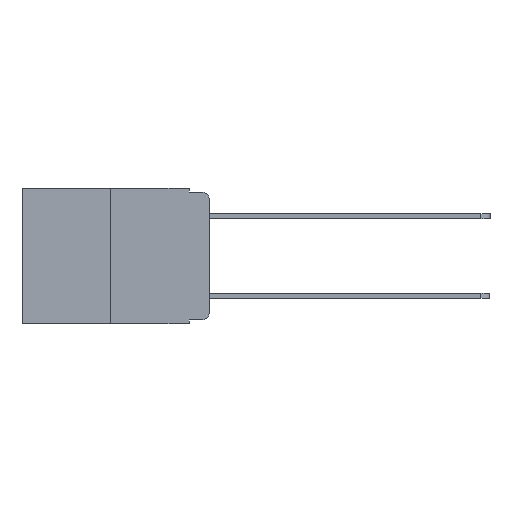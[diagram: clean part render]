
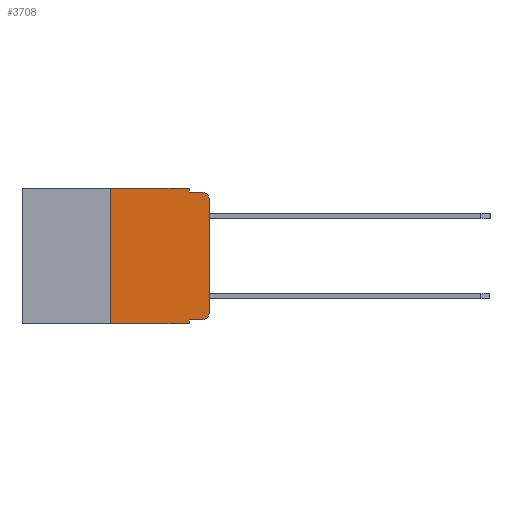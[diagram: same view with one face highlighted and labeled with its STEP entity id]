
A CAD part, left-side view. The second image highlights one B-rep face of the part: STEP entity #3708.
In plain terms, the highlighted planar face has unit normal (-1, 0, 0).
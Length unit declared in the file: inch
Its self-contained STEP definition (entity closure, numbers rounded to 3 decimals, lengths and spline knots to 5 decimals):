
#12 = EDGE_CURVE ( 'NONE', #16790, #11904, #22205, .T. ) ;
#94 = CARTESIAN_POINT ( 'NONE',  ( 0., 0., -0.313 ) ) ;
#160 = FACE_OUTER_BOUND ( 'NONE', #13219, .T. ) ;
#509 = EDGE_CURVE ( 'NONE', #11904, #1297, #18472, .T. ) ;
#678 = DIRECTION ( 'NONE',  ( 0., 0., -1. ) ) ;
#687 = CARTESIAN_POINT ( 'NONE',  ( 0., 0.25, 0. ) ) ;
#1297 = VERTEX_POINT ( 'NONE', #94 ) ;
#1378 = CARTESIAN_POINT ( 'NONE',  ( 0., 0.02, -0.01 ) ) ;
#1591 = ORIENTED_EDGE ( 'NONE', *, *, #10292, .T. ) ;
#1808 = CARTESIAN_POINT ( 'NONE',  ( 0., 0.473, 0. ) ) ;
#3054 = CARTESIAN_POINT ( 'NONE',  ( 0., 0.051, 0. ) ) ;
#3351 = CARTESIAN_POINT ( 'NONE',  ( 0., 0.051, -0.343 ) ) ;
#3483 = VECTOR ( 'NONE', #13661, 39.37008 ) ;
#3509 = DIRECTION ( 'NONE',  ( 0., 0., -1. ) ) ;
#3539 = DIRECTION ( 'NONE',  ( -1., 0., 0. ) ) ;
#3667 = CARTESIAN_POINT ( 'NONE',  ( 0., 0.051, 0. ) ) ;
#3708 = ADVANCED_FACE ( 'NONE', ( #160 ), #17959, .F. ) ;
#3719 = DIRECTION ( 'NONE',  ( 0., -1., 0. ) ) ;
#4081 = LINE ( 'NONE', #687, #3483 ) ;
#4088 = LINE ( 'NONE', #3054, #18382 ) ;
#4102 = LINE ( 'NONE', #4581, #22365 ) ;
#4274 = ORIENTED_EDGE ( 'NONE', *, *, #8604, .F. ) ;
#4296 = DIRECTION ( 'NONE',  ( 0., -1., 0. ) ) ;
#4581 = CARTESIAN_POINT ( 'NONE',  ( 0., 0., 0. ) ) ;
#5077 = CARTESIAN_POINT ( 'NONE',  ( 0., 0.051, -0.333 ) ) ;
#5721 = ORIENTED_EDGE ( 'NONE', *, *, #20432, .T. ) ;
#5916 = EDGE_CURVE ( 'NONE', #13882, #7065, #23062, .T. ) ;
#6126 = CARTESIAN_POINT ( 'NONE',  ( 0., 0.25, -0.343 ) ) ;
#6276 = VECTOR ( 'NONE', #10702, 39.37008 ) ;
#7065 = VERTEX_POINT ( 'NONE', #3667 ) ;
#7349 = DIRECTION ( 'NONE',  ( 0., 0., -1. ) ) ;
#7488 = ORIENTED_EDGE ( 'NONE', *, *, #13862, .T. ) ;
#7541 = VERTEX_POINT ( 'NONE', #15515 ) ;
#8204 = CARTESIAN_POINT ( 'NONE',  ( 0., 0.25, 0. ) ) ;
#8300 = VECTOR ( 'NONE', #21865, 39.37008 ) ;
#8604 = EDGE_CURVE ( 'NONE', #7065, #7541, #4088, .T. ) ;
#9168 = CARTESIAN_POINT ( 'NONE',  ( 0., 0.473, 0. ) ) ;
#9256 = ORIENTED_EDGE ( 'NONE', *, *, #5916, .F. ) ;
#9289 = VECTOR ( 'NONE', #3719, 39.37008 ) ;
#9515 = LINE ( 'NONE', #15171, #18799 ) ;
#10292 = EDGE_CURVE ( 'NONE', #20953, #23064, #9515, .T. ) ;
#10702 = DIRECTION ( 'NONE',  ( 0., -1., 0. ) ) ;
#11309 = AXIS2_PLACEMENT_3D ( 'NONE', #22149, #11958, #678 ) ;
#11904 = VERTEX_POINT ( 'NONE', #21791 ) ;
#11958 = DIRECTION ( 'NONE',  ( -1., 0., 0. ) ) ;
#12149 = DIRECTION ( 'NONE',  ( 0., 0., 1. ) ) ;
#12350 = CARTESIAN_POINT ( 'NONE',  ( 0., 0.051, 0. ) ) ;
#12417 = DIRECTION ( 'NONE',  ( 0., 0., -1. ) ) ;
#12805 = DIRECTION ( 'NONE',  ( 1., 0., 0. ) ) ;
#13219 = EDGE_LOOP ( 'NONE', ( #5721, #7488, #16939, #4274, #9256, #23029, #1591, #16678, #17758, #13724 ) ) ;
#13661 = DIRECTION ( 'NONE',  ( 0., 0., 1. ) ) ;
#13724 = ORIENTED_EDGE ( 'NONE', *, *, #509, .T. ) ;
#13862 = EDGE_CURVE ( 'NONE', #16828, #15884, #21467, .T. ) ;
#13882 = VERTEX_POINT ( 'NONE', #8204 ) ;
#14011 = DIRECTION ( 'NONE',  ( 0., 0., -1. ) ) ;
#14918 = CARTESIAN_POINT ( 'NONE',  ( 0., 0., -0.03 ) ) ;
#15019 = EDGE_CURVE ( 'NONE', #7541, #15884, #20357, .T. ) ;
#15171 = CARTESIAN_POINT ( 'NONE',  ( 0., 0.473, -0.343 ) ) ;
#15441 = VECTOR ( 'NONE', #12417, 39.37008 ) ;
#15515 = CARTESIAN_POINT ( 'NONE',  ( 0., 0.051, -0.01 ) ) ;
#15884 = VERTEX_POINT ( 'NONE', #1378 ) ;
#16678 = ORIENTED_EDGE ( 'NONE', *, *, #18037, .F. ) ;
#16790 = VERTEX_POINT ( 'NONE', #18223 ) ;
#16828 = VERTEX_POINT ( 'NONE', #14918 ) ;
#16939 = ORIENTED_EDGE ( 'NONE', *, *, #15019, .F. ) ;
#17051 = AXIS2_PLACEMENT_3D ( 'NONE', #9168, #12805, #7349 ) ;
#17450 = CARTESIAN_POINT ( 'NONE',  ( 0., 0.02, -0.313 ) ) ;
#17758 = ORIENTED_EDGE ( 'NONE', *, *, #12, .T. ) ;
#17959 = PLANE ( 'NONE',  #17051 ) ;
#18037 = EDGE_CURVE ( 'NONE', #16790, #23064, #19977, .T. ) ;
#18223 = CARTESIAN_POINT ( 'NONE',  ( 0., 0.051, -0.333 ) ) ;
#18382 = VECTOR ( 'NONE', #14011, 39.37008 ) ;
#18472 = CIRCLE ( 'NONE', #19101, 0.02 ) ;
#18799 = VECTOR ( 'NONE', #4296, 39.37008 ) ;
#19101 = AXIS2_PLACEMENT_3D ( 'NONE', #17450, #3539, #3509 ) ;
#19306 = CARTESIAN_POINT ( 'NONE',  ( 0., 0.051, -0.01 ) ) ;
#19977 = LINE ( 'NONE', #12350, #15441 ) ;
#20357 = LINE ( 'NONE', #19306, #6276 ) ;
#20432 = EDGE_CURVE ( 'NONE', #1297, #16828, #4102, .T. ) ;
#20953 = VERTEX_POINT ( 'NONE', #6126 ) ;
#21467 = CIRCLE ( 'NONE', #11309, 0.02 ) ;
#21791 = CARTESIAN_POINT ( 'NONE',  ( 0., 0.02, -0.333 ) ) ;
#21857 = EDGE_CURVE ( 'NONE', #20953, #13882, #4081, .T. ) ;
#21865 = DIRECTION ( 'NONE',  ( 0., -1., 0. ) ) ;
#22149 = CARTESIAN_POINT ( 'NONE',  ( 0., 0.02, -0.03 ) ) ;
#22205 = LINE ( 'NONE', #5077, #8300 ) ;
#22365 = VECTOR ( 'NONE', #12149, 39.37008 ) ;
#23029 = ORIENTED_EDGE ( 'NONE', *, *, #21857, .F. ) ;
#23062 = LINE ( 'NONE', #1808, #9289 ) ;
#23064 = VERTEX_POINT ( 'NONE', #3351 ) ;
